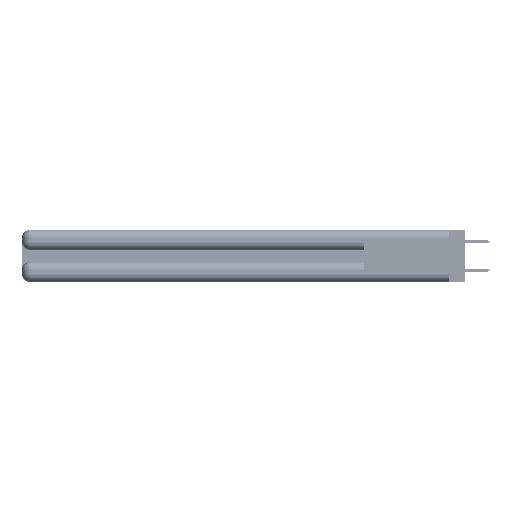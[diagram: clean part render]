
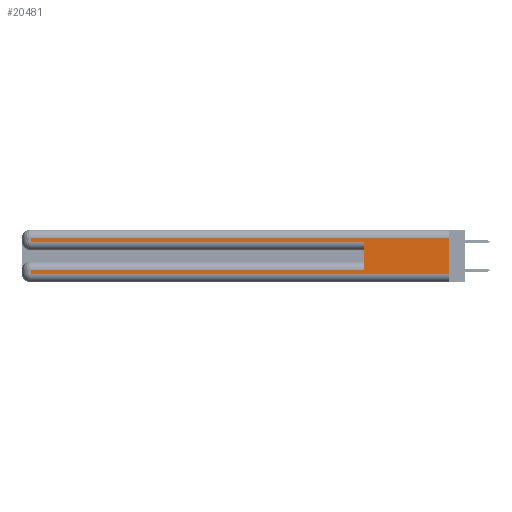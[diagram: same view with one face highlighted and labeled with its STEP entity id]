
A CAD part, left-side view. The second image highlights one B-rep face of the part: STEP entity #20481.
In plain terms, the highlighted planar face has unit normal (-1, 0, 0).
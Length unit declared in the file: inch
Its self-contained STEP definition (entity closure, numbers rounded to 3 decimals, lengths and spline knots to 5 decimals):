
#850 = DIRECTION ( 'NONE',  ( 0., 0., -1. ) ) ;
#1065 = DIRECTION ( 'NONE',  ( 0., -1., 0. ) ) ;
#1202 = LINE ( 'NONE', #27015, #34216 ) ;
#1285 = VERTEX_POINT ( 'NONE', #41807 ) ;
#4186 = EDGE_CURVE ( 'NONE', #52343, #50835, #7059, .T. ) ;
#5299 = VECTOR ( 'NONE', #1065, 39.37008 ) ;
#6319 = ORIENTED_EDGE ( 'NONE', *, *, #12758, .T. ) ;
#7059 = LINE ( 'NONE', #50702, #9100 ) ;
#8191 = ORIENTED_EDGE ( 'NONE', *, *, #42005, .F. ) ;
#8756 = CARTESIAN_POINT ( 'NONE',  ( 0., 2.94, 0.37 ) ) ;
#9100 = VECTOR ( 'NONE', #49414, 39.37008 ) ;
#9488 = VECTOR ( 'NONE', #44612, 39.37008 ) ;
#9983 = EDGE_CURVE ( 'NONE', #52222, #14186, #42143, .T. ) ;
#10478 = CARTESIAN_POINT ( 'NONE',  ( 0., 0.6, 0.085 ) ) ;
#10865 = CARTESIAN_POINT ( 'NONE',  ( 0., 0., 0.085 ) ) ;
#11724 = CARTESIAN_POINT ( 'NONE',  ( 0., 0., 0.285 ) ) ;
#11924 = EDGE_LOOP ( 'NONE', ( #8191, #48138, #47901, #29984, #16720, #38742, #19214, #6319 ) ) ;
#12758 = EDGE_CURVE ( 'NONE', #50717, #1285, #15201, .T. ) ;
#13118 = CARTESIAN_POINT ( 'NONE',  ( 0., 2.94, 0.06 ) ) ;
#14186 = VERTEX_POINT ( 'NONE', #38765 ) ;
#14387 = EDGE_CURVE ( 'NONE', #40436, #14186, #24895, .T. ) ;
#15201 = LINE ( 'NONE', #43287, #5299 ) ;
#16720 = ORIENTED_EDGE ( 'NONE', *, *, #9983, .F. ) ;
#17727 = DIRECTION ( 'NONE',  ( 0., 0., 1. ) ) ;
#19214 = ORIENTED_EDGE ( 'NONE', *, *, #41646, .T. ) ;
#19691 = CARTESIAN_POINT ( 'NONE',  ( 0., 0., 0.31 ) ) ;
#20481 = ADVANCED_FACE ( 'NONE', ( #27333 ), #21612, .F. ) ;
#20720 = LINE ( 'NONE', #10865, #9488 ) ;
#21086 = CARTESIAN_POINT ( 'NONE',  ( 0., 0., 0.37 ) ) ;
#21612 = PLANE ( 'NONE',  #43772 ) ;
#22336 = CARTESIAN_POINT ( 'NONE',  ( 0., 0., 0.37 ) ) ;
#24895 = LINE ( 'NONE', #11724, #36141 ) ;
#27015 = CARTESIAN_POINT ( 'NONE',  ( 0., 2.94, 0.37 ) ) ;
#27333 = FACE_OUTER_BOUND ( 'NONE', #11924, .T. ) ;
#28284 = LINE ( 'NONE', #8756, #44066 ) ;
#29984 = ORIENTED_EDGE ( 'NONE', *, *, #14387, .T. ) ;
#31462 = VERTEX_POINT ( 'NONE', #37218 ) ;
#33182 = EDGE_CURVE ( 'NONE', #52222, #31462, #20720, .T. ) ;
#33475 = DIRECTION ( 'NONE',  ( 0., 0., -1. ) ) ;
#34216 = VECTOR ( 'NONE', #47508, 39.37008 ) ;
#35595 = VECTOR ( 'NONE', #33475, 39.37008 ) ;
#36141 = VECTOR ( 'NONE', #41225, 39.37008 ) ;
#37218 = CARTESIAN_POINT ( 'NONE',  ( 0., 2.94, 0.085 ) ) ;
#38742 = ORIENTED_EDGE ( 'NONE', *, *, #33182, .T. ) ;
#38765 = CARTESIAN_POINT ( 'NONE',  ( 0., 0.6, 0.285 ) ) ;
#40436 = VERTEX_POINT ( 'NONE', #46711 ) ;
#41225 = DIRECTION ( 'NONE',  ( 0., -1., 0. ) ) ;
#41479 = LINE ( 'NONE', #21086, #35595 ) ;
#41646 = EDGE_CURVE ( 'NONE', #31462, #50717, #28284, .T. ) ;
#41767 = EDGE_CURVE ( 'NONE', #50835, #40436, #1202, .T. ) ;
#41807 = CARTESIAN_POINT ( 'NONE',  ( 0., 0., 0.06 ) ) ;
#42005 = EDGE_CURVE ( 'NONE', #52343, #1285, #41479, .T. ) ;
#42143 = LINE ( 'NONE', #42609, #50743 ) ;
#42609 = CARTESIAN_POINT ( 'NONE',  ( 0., 0.6, 0.145 ) ) ;
#43287 = CARTESIAN_POINT ( 'NONE',  ( 0., 0., 0.06 ) ) ;
#43772 = AXIS2_PLACEMENT_3D ( 'NONE', #22336, #51514, #51146 ) ;
#44066 = VECTOR ( 'NONE', #850, 39.37008 ) ;
#44612 = DIRECTION ( 'NONE',  ( 0., 1., 0. ) ) ;
#46711 = CARTESIAN_POINT ( 'NONE',  ( 0., 2.94, 0.285 ) ) ;
#47508 = DIRECTION ( 'NONE',  ( 0., 0., -1. ) ) ;
#47901 = ORIENTED_EDGE ( 'NONE', *, *, #41767, .T. ) ;
#48138 = ORIENTED_EDGE ( 'NONE', *, *, #4186, .T. ) ;
#49414 = DIRECTION ( 'NONE',  ( 0., 1., 0. ) ) ;
#50702 = CARTESIAN_POINT ( 'NONE',  ( 0., 0., 0.31 ) ) ;
#50717 = VERTEX_POINT ( 'NONE', #13118 ) ;
#50743 = VECTOR ( 'NONE', #17727, 39.37008 ) ;
#50835 = VERTEX_POINT ( 'NONE', #51504 ) ;
#51146 = DIRECTION ( 'NONE',  ( 0., 0., -1. ) ) ;
#51504 = CARTESIAN_POINT ( 'NONE',  ( 0., 2.94, 0.31 ) ) ;
#51514 = DIRECTION ( 'NONE',  ( 1., 0., 0. ) ) ;
#52222 = VERTEX_POINT ( 'NONE', #10478 ) ;
#52343 = VERTEX_POINT ( 'NONE', #19691 ) ;
